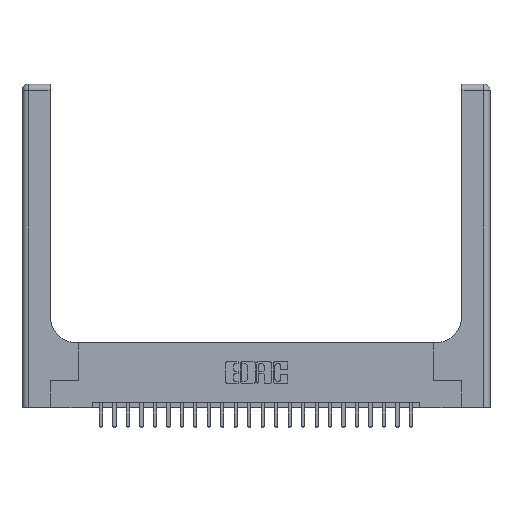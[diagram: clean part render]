
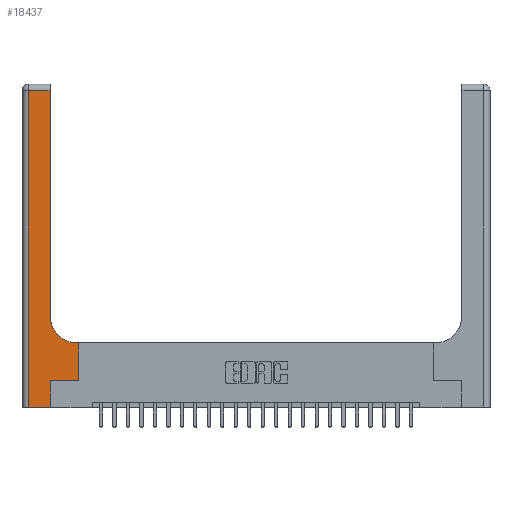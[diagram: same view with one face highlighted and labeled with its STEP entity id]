
A CAD part, top view. The second image highlights one B-rep face of the part: STEP entity #18437.
In plain terms, the highlighted planar face has unit normal (0, 0, 1).
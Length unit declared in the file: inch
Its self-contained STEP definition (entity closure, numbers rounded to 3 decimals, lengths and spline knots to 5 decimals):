
#750 = CARTESIAN_POINT ( 'NONE',  ( 0.26, 0.6, 0.37 ) ) ;
#1586 = ORIENTED_EDGE ( 'NONE', *, *, #16632, .T. ) ;
#2354 = VERTEX_POINT ( 'NONE', #18569 ) ;
#2462 = VERTEX_POINT ( 'NONE', #21966 ) ;
#2511 = AXIS2_PLACEMENT_3D ( 'NONE', #23626, #16362, #5631 ) ;
#2810 = ORIENTED_EDGE ( 'NONE', *, *, #9567, .T. ) ;
#3051 = VECTOR ( 'NONE', #3624, 39.37008 ) ;
#3101 = FACE_OUTER_BOUND ( 'NONE', #19470, .T. ) ;
#3562 = LINE ( 'NONE', #7055, #10961 ) ;
#3624 = DIRECTION ( 'NONE',  ( 1., 0., 0. ) ) ;
#3808 = DIRECTION ( 'NONE',  ( 0., 1., 0. ) ) ;
#3985 = ORIENTED_EDGE ( 'NONE', *, *, #12814, .T. ) ;
#4097 = VECTOR ( 'NONE', #5502, 39.37008 ) ;
#4148 = VERTEX_POINT ( 'NONE', #10003 ) ;
#4159 = CARTESIAN_POINT ( 'NONE',  ( 0., 2.94, 0.37 ) ) ;
#4340 = ORIENTED_EDGE ( 'NONE', *, *, #8460, .T. ) ;
#4666 = CARTESIAN_POINT ( 'NONE',  ( 0.06, 2.94, 0.37 ) ) ;
#4941 = VECTOR ( 'NONE', #3808, 39.37008 ) ;
#5502 = DIRECTION ( 'NONE',  ( 0., 1., 0. ) ) ;
#5631 = DIRECTION ( 'NONE',  ( 1., 0., 0. ) ) ;
#5643 = LINE ( 'NONE', #18554, #4097 ) ;
#5727 = VECTOR ( 'NONE', #22284, 39.37008 ) ;
#5994 = CARTESIAN_POINT ( 'NONE',  ( 0.26, 0.85, 0.37 ) ) ;
#6465 = EDGE_CURVE ( 'NONE', #2354, #9745, #9832, .T. ) ;
#6867 = DIRECTION ( 'NONE',  ( 1., 0., 0. ) ) ;
#7055 = CARTESIAN_POINT ( 'NONE',  ( 0.26, 3., 0.37 ) ) ;
#7184 = CARTESIAN_POINT ( 'NONE',  ( 0.06, 3., 0.37 ) ) ;
#7399 = CARTESIAN_POINT ( 'NONE',  ( 0.265, 0.25, 0.37 ) ) ;
#7400 = CARTESIAN_POINT ( 'NONE',  ( 0.528, 0.25, 0.37 ) ) ;
#8150 = ORIENTED_EDGE ( 'NONE', *, *, #15366, .T. ) ;
#8404 = DIRECTION ( 'NONE',  ( 0., 0., -1. ) ) ;
#8406 = CARTESIAN_POINT ( 'NONE',  ( 0.26, 2.94, 0.37 ) ) ;
#8460 = EDGE_CURVE ( 'NONE', #15622, #11237, #11532, .T. ) ;
#8659 = ORIENTED_EDGE ( 'NONE', *, *, #12842, .T. ) ;
#9567 = EDGE_CURVE ( 'NONE', #4148, #2354, #15787, .T. ) ;
#9745 = VERTEX_POINT ( 'NONE', #5994 ) ;
#9832 = CIRCLE ( 'NONE', #2511, 0.25 ) ;
#10003 = CARTESIAN_POINT ( 'NONE',  ( 0.528, 0.6, 0.37 ) ) ;
#10264 = AXIS2_PLACEMENT_3D ( 'NONE', #17687, #8404, #10443 ) ;
#10443 = DIRECTION ( 'NONE',  ( -1., 0., 0. ) ) ;
#10591 = EDGE_CURVE ( 'NONE', #11565, #2462, #21981, .T. ) ;
#10915 = DIRECTION ( 'NONE',  ( 0., 1., 0. ) ) ;
#10961 = VECTOR ( 'NONE', #10915, 39.37008 ) ;
#11010 = EDGE_CURVE ( 'NONE', #20137, #21930, #14568, .T. ) ;
#11237 = VERTEX_POINT ( 'NONE', #4666 ) ;
#11532 = LINE ( 'NONE', #4159, #16348 ) ;
#11565 = VERTEX_POINT ( 'NONE', #18646 ) ;
#12814 = EDGE_CURVE ( 'NONE', #11237, #11565, #14637, .T. ) ;
#12842 = EDGE_CURVE ( 'NONE', #2462, #20137, #20469, .T. ) ;
#13459 = DIRECTION ( 'NONE',  ( -1., 0., 0. ) ) ;
#14024 = VECTOR ( 'NONE', #17602, 39.37008 ) ;
#14568 = LINE ( 'NONE', #23413, #14991 ) ;
#14637 = LINE ( 'NONE', #7184, #5727 ) ;
#14991 = VECTOR ( 'NONE', #6867, 39.37008 ) ;
#15366 = EDGE_CURVE ( 'NONE', #21930, #4148, #5643, .T. ) ;
#15622 = VERTEX_POINT ( 'NONE', #8406 ) ;
#15761 = PLANE ( 'NONE',  #10264 ) ;
#15787 = LINE ( 'NONE', #750, #14024 ) ;
#16348 = VECTOR ( 'NONE', #13459, 39.37008 ) ;
#16362 = DIRECTION ( 'NONE',  ( 0., 0., -1. ) ) ;
#16632 = EDGE_CURVE ( 'NONE', #9745, #15622, #3562, .T. ) ;
#17602 = DIRECTION ( 'NONE',  ( -1., 0., 0. ) ) ;
#17687 = CARTESIAN_POINT ( 'NONE',  ( 0., 3., 0.37 ) ) ;
#18437 = ADVANCED_FACE ( 'NONE', ( #3101 ), #15761, .F. ) ;
#18554 = CARTESIAN_POINT ( 'NONE',  ( 0.528, 0.25, 0.37 ) ) ;
#18569 = CARTESIAN_POINT ( 'NONE',  ( 0.51, 0.6, 0.37 ) ) ;
#18646 = CARTESIAN_POINT ( 'NONE',  ( 0.06, 0., 0.37 ) ) ;
#18810 = ORIENTED_EDGE ( 'NONE', *, *, #11010, .T. ) ;
#19419 = ORIENTED_EDGE ( 'NONE', *, *, #6465, .T. ) ;
#19470 = EDGE_LOOP ( 'NONE', ( #1586, #4340, #3985, #23587, #8659, #18810, #8150, #2810, #19419 ) ) ;
#20137 = VERTEX_POINT ( 'NONE', #7399 ) ;
#20469 = LINE ( 'NONE', #22026, #4941 ) ;
#21930 = VERTEX_POINT ( 'NONE', #7400 ) ;
#21966 = CARTESIAN_POINT ( 'NONE',  ( 0.265, 0., 0.37 ) ) ;
#21981 = LINE ( 'NONE', #23664, #3051 ) ;
#22026 = CARTESIAN_POINT ( 'NONE',  ( 0.265, 0., 0.37 ) ) ;
#22284 = DIRECTION ( 'NONE',  ( 0., -1., 0. ) ) ;
#23413 = CARTESIAN_POINT ( 'NONE',  ( 0.265, 0.25, 0.37 ) ) ;
#23587 = ORIENTED_EDGE ( 'NONE', *, *, #10591, .T. ) ;
#23626 = CARTESIAN_POINT ( 'NONE',  ( 0.51, 0.85, 0.37 ) ) ;
#23664 = CARTESIAN_POINT ( 'NONE',  ( 0., 0., 0.37 ) ) ;
